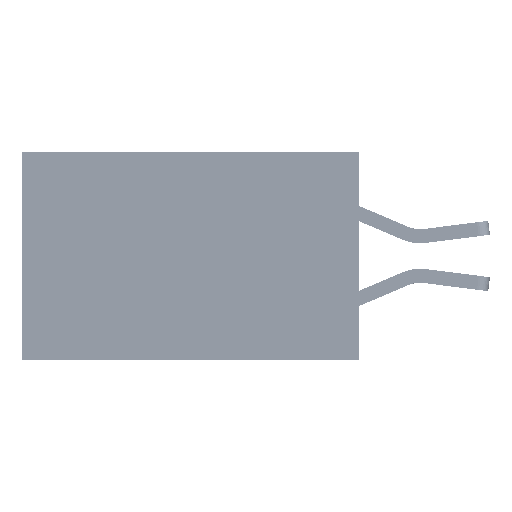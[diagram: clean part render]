
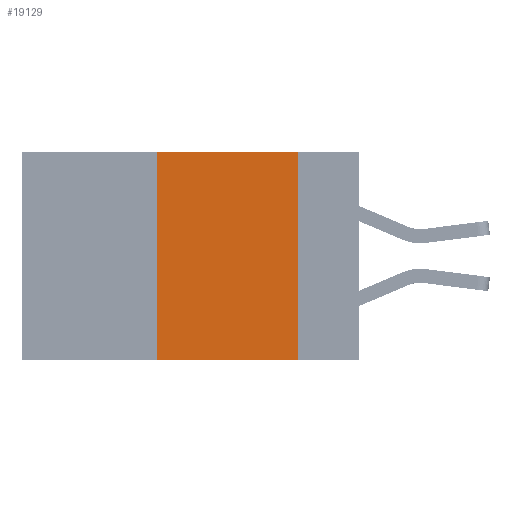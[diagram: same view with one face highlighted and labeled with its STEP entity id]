
A CAD part, left-side view. The second image highlights one B-rep face of the part: STEP entity #19129.
In plain terms, the highlighted planar face has unit normal (-1, 0, 0).
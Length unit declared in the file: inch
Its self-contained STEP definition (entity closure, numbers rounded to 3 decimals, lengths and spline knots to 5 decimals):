
#1428 = CARTESIAN_POINT ( 'NONE',  ( 0., 0.11, 0. ) ) ;
#3755 = VERTEX_POINT ( 'NONE', #31701 ) ;
#4419 = ORIENTED_EDGE ( 'NONE', *, *, #41898, .F. ) ;
#5331 = EDGE_CURVE ( 'NONE', #34784, #21951, #45271, .T. ) ;
#6000 = PLANE ( 'NONE',  #37357 ) ;
#6333 = CARTESIAN_POINT ( 'NONE',  ( 0., 0.11, -0.37 ) ) ;
#8347 = ORIENTED_EDGE ( 'NONE', *, *, #29557, .F. ) ;
#10515 = VECTOR ( 'NONE', #43698, 39.37008 ) ;
#13631 = DIRECTION ( 'NONE',  ( 1., 0., 0. ) ) ;
#14584 = LINE ( 'NONE', #34109, #27652 ) ;
#16175 = DIRECTION ( 'NONE',  ( 0., 0., 1. ) ) ;
#19129 = ADVANCED_FACE ( 'NONE', ( #28854 ), #6000, .F. ) ;
#21823 = VECTOR ( 'NONE', #26844, 39.37008 ) ;
#21951 = VERTEX_POINT ( 'NONE', #6333 ) ;
#22402 = VERTEX_POINT ( 'NONE', #41734 ) ;
#23056 = EDGE_LOOP ( 'NONE', ( #35136, #8347, #4419, #35998 ) ) ;
#24670 = LINE ( 'NONE', #1428, #21823 ) ;
#26321 = LINE ( 'NONE', #41427, #46825 ) ;
#26844 = DIRECTION ( 'NONE',  ( 0., 0., -1. ) ) ;
#27652 = VECTOR ( 'NONE', #16175, 39.37008 ) ;
#28559 = CARTESIAN_POINT ( 'NONE',  ( 0., 0.6, -0.37 ) ) ;
#28854 = FACE_OUTER_BOUND ( 'NONE', #23056, .T. ) ;
#29557 = EDGE_CURVE ( 'NONE', #22402, #3755, #26321, .T. ) ;
#31428 = CARTESIAN_POINT ( 'NONE',  ( 0., 0.6, 0. ) ) ;
#31701 = CARTESIAN_POINT ( 'NONE',  ( 0., 0.11, 0. ) ) ;
#32480 = CARTESIAN_POINT ( 'NONE',  ( 0., 0.36, -0.37 ) ) ;
#34109 = CARTESIAN_POINT ( 'NONE',  ( 0., 0.36, 0. ) ) ;
#34784 = VERTEX_POINT ( 'NONE', #32480 ) ;
#35136 = ORIENTED_EDGE ( 'NONE', *, *, #35649, .F. ) ;
#35649 = EDGE_CURVE ( 'NONE', #3755, #21951, #24670, .T. ) ;
#35998 = ORIENTED_EDGE ( 'NONE', *, *, #5331, .T. ) ;
#37357 = AXIS2_PLACEMENT_3D ( 'NONE', #31428, #13631, #46404 ) ;
#38076 = DIRECTION ( 'NONE',  ( 0., -1., 0. ) ) ;
#41427 = CARTESIAN_POINT ( 'NONE',  ( 0., 0.6, 0. ) ) ;
#41734 = CARTESIAN_POINT ( 'NONE',  ( 0., 0.36, 0. ) ) ;
#41898 = EDGE_CURVE ( 'NONE', #34784, #22402, #14584, .T. ) ;
#43698 = DIRECTION ( 'NONE',  ( 0., -1., 0. ) ) ;
#45271 = LINE ( 'NONE', #28559, #10515 ) ;
#46404 = DIRECTION ( 'NONE',  ( 0., 0., -1. ) ) ;
#46825 = VECTOR ( 'NONE', #38076, 39.37008 ) ;
